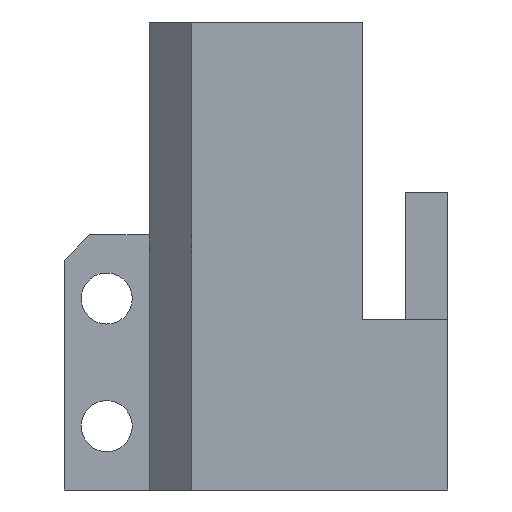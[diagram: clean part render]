
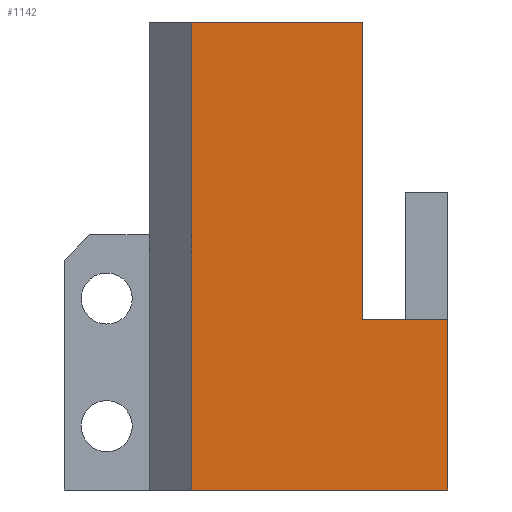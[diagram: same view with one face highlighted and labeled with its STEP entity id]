
A CAD part, left-side view. The second image highlights one B-rep face of the part: STEP entity #1142.
In plain terms, the highlighted planar face has unit normal (-1, 0, 0).
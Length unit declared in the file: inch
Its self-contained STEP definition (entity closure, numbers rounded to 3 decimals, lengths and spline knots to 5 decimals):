
#17 = VECTOR ( 'NONE', #940, 39.37008 ) ;
#19 = ORIENTED_EDGE ( 'NONE', *, *, #70, .T. ) ;
#32 = VECTOR ( 'NONE', #186, 39.37008 ) ;
#34 = VERTEX_POINT ( 'NONE', #546 ) ;
#70 = EDGE_CURVE ( 'NONE', #1070, #388, #987, .T. ) ;
#89 = ORIENTED_EDGE ( 'NONE', *, *, #262, .T. ) ;
#118 = EDGE_CURVE ( 'NONE', #827, #1070, #746, .T. ) ;
#122 = DIRECTION ( 'NONE',  ( 1., 0., 0. ) ) ;
#125 = ORIENTED_EDGE ( 'NONE', *, *, #217, .F. ) ;
#129 = AXIS2_PLACEMENT_3D ( 'NONE', #469, #122, #937 ) ;
#133 = DIRECTION ( 'NONE',  ( 0., 0., 1. ) ) ;
#170 = CARTESIAN_POINT ( 'NONE',  ( -2.235, 2.00996, -2. ) ) ;
#186 = DIRECTION ( 'NONE',  ( 0., 0., -1. ) ) ;
#201 = LINE ( 'NONE', #646, #17 ) ;
#216 = VECTOR ( 'NONE', #1162, 39.37008 ) ;
#217 = EDGE_CURVE ( 'NONE', #355, #388, #669, .T. ) ;
#235 = CARTESIAN_POINT ( 'NONE',  ( -2.235, -1., 0. ) ) ;
#262 = EDGE_CURVE ( 'NONE', #355, #34, #649, .T. ) ;
#266 = CARTESIAN_POINT ( 'NONE',  ( -2.235, 2.00996, 3.5 ) ) ;
#272 = CARTESIAN_POINT ( 'NONE',  ( -2.235, -1., -2. ) ) ;
#292 = FACE_OUTER_BOUND ( 'NONE', #938, .T. ) ;
#332 = DIRECTION ( 'NONE',  ( 0., -1., 0. ) ) ;
#355 = VERTEX_POINT ( 'NONE', #266 ) ;
#379 = LINE ( 'NONE', #272, #32 ) ;
#387 = VECTOR ( 'NONE', #959, 39.37008 ) ;
#388 = VERTEX_POINT ( 'NONE', #643 ) ;
#417 = CARTESIAN_POINT ( 'NONE',  ( -2.235, -1., -2. ) ) ;
#469 = CARTESIAN_POINT ( 'NONE',  ( -2.235, 0., -2. ) ) ;
#487 = EDGE_CURVE ( 'NONE', #827, #786, #379, .T. ) ;
#529 = EDGE_CURVE ( 'NONE', #786, #34, #201, .T. ) ;
#546 = CARTESIAN_POINT ( 'NONE',  ( -2.235, 2.00996, -2. ) ) ;
#550 = ORIENTED_EDGE ( 'NONE', *, *, #529, .F. ) ;
#580 = ORIENTED_EDGE ( 'NONE', *, *, #487, .F. ) ;
#643 = CARTESIAN_POINT ( 'NONE',  ( -2.235, 0., 3.5 ) ) ;
#646 = CARTESIAN_POINT ( 'NONE',  ( -2.235, 0., -2. ) ) ;
#649 = LINE ( 'NONE', #170, #216 ) ;
#669 = LINE ( 'NONE', #876, #1001 ) ;
#746 = LINE ( 'NONE', #235, #387 ) ;
#786 = VERTEX_POINT ( 'NONE', #417 ) ;
#827 = VERTEX_POINT ( 'NONE', #1064 ) ;
#872 = VECTOR ( 'NONE', #133, 39.37008 ) ;
#876 = CARTESIAN_POINT ( 'NONE',  ( -2.235, 0., 3.5 ) ) ;
#909 = ORIENTED_EDGE ( 'NONE', *, *, #118, .T. ) ;
#931 = PLANE ( 'NONE',  #129 ) ;
#937 = DIRECTION ( 'NONE',  ( 0., 0., -1. ) ) ;
#938 = EDGE_LOOP ( 'NONE', ( #125, #89, #550, #580, #909, #19 ) ) ;
#940 = DIRECTION ( 'NONE',  ( 0., 1., 0. ) ) ;
#959 = DIRECTION ( 'NONE',  ( 0., 1., 0. ) ) ;
#987 = LINE ( 'NONE', #1044, #872 ) ;
#1001 = VECTOR ( 'NONE', #332, 39.37008 ) ;
#1002 = CARTESIAN_POINT ( 'NONE',  ( -2.235, 0., 0. ) ) ;
#1044 = CARTESIAN_POINT ( 'NONE',  ( -2.235, 0., -2. ) ) ;
#1064 = CARTESIAN_POINT ( 'NONE',  ( -2.235, -1., 0. ) ) ;
#1070 = VERTEX_POINT ( 'NONE', #1002 ) ;
#1142 = ADVANCED_FACE ( 'NONE', ( #292 ), #931, .F. ) ;
#1162 = DIRECTION ( 'NONE',  ( 0., 0., -1. ) ) ;
